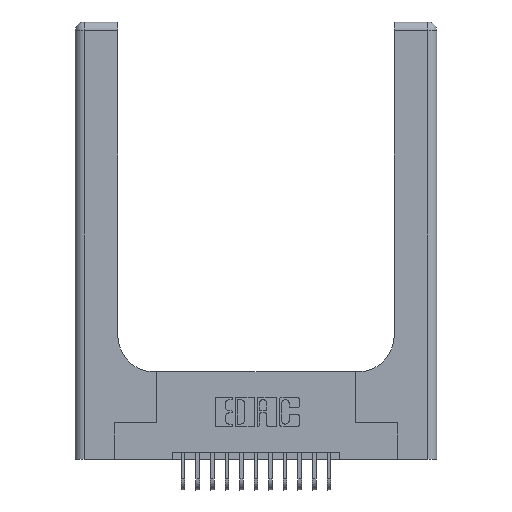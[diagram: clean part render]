
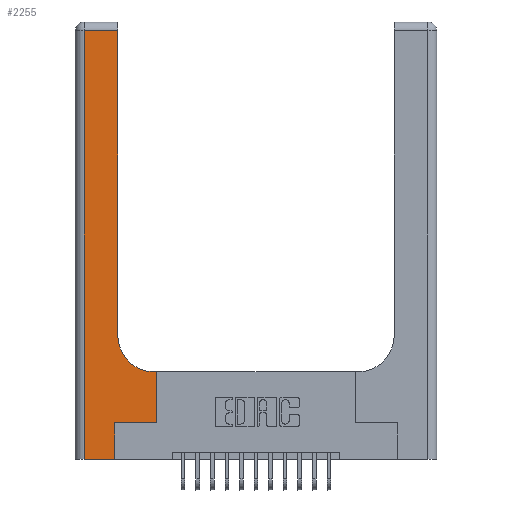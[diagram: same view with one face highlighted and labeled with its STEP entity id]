
A CAD part, top view. The second image highlights one B-rep face of the part: STEP entity #2255.
In plain terms, the highlighted planar face has unit normal (0, 0, 1).
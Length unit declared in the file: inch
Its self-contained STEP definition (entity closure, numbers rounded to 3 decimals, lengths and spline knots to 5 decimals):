
#16 = VECTOR ( 'NONE', #14650, 39.37008 ) ;
#602 = LINE ( 'NONE', #11856, #10853 ) ;
#679 = DIRECTION ( 'NONE',  ( 0., 0., -1. ) ) ;
#1124 = CARTESIAN_POINT ( 'NONE',  ( 0.269, 0., 0.37 ) ) ;
#1543 = DIRECTION ( 'NONE',  ( 0., 1., 0. ) ) ;
#1904 = CARTESIAN_POINT ( 'NONE',  ( 0.5585, 0.6, 0.37 ) ) ;
#1957 = LINE ( 'NONE', #9040, #16 ) ;
#2153 = EDGE_CURVE ( 'NONE', #2332, #11790, #8864, .T. ) ;
#2218 = VECTOR ( 'NONE', #12598, 39.37008 ) ;
#2237 = DIRECTION ( 'NONE',  ( 1., 0., 0. ) ) ;
#2255 = ADVANCED_FACE ( 'NONE', ( #17376 ), #9084, .F. ) ;
#2332 = VERTEX_POINT ( 'NONE', #1904 ) ;
#2705 = LINE ( 'NONE', #9562, #2218 ) ;
#3342 = VERTEX_POINT ( 'NONE', #10067 ) ;
#3783 = VECTOR ( 'NONE', #17413, 39.37008 ) ;
#3848 = EDGE_CURVE ( 'NONE', #3342, #5929, #4271, .T. ) ;
#3990 = ORIENTED_EDGE ( 'NONE', *, *, #2153, .T. ) ;
#4271 = LINE ( 'NONE', #15719, #3783 ) ;
#4307 = CIRCLE ( 'NONE', #9821, 0.25 ) ;
#4372 = DIRECTION ( 'NONE',  ( 0., 0., -1. ) ) ;
#5025 = CARTESIAN_POINT ( 'NONE',  ( 0.06, 2.94, 0.37 ) ) ;
#5256 = ORIENTED_EDGE ( 'NONE', *, *, #3848, .T. ) ;
#5929 = VERTEX_POINT ( 'NONE', #1124 ) ;
#6102 = EDGE_CURVE ( 'NONE', #5929, #15019, #13460, .T. ) ;
#6282 = VERTEX_POINT ( 'NONE', #5025 ) ;
#7884 = EDGE_CURVE ( 'NONE', #10802, #2332, #602, .T. ) ;
#8006 = ORIENTED_EDGE ( 'NONE', *, *, #7884, .T. ) ;
#8408 = LINE ( 'NONE', #17458, #19035 ) ;
#8812 = VERTEX_POINT ( 'NONE', #16460 ) ;
#8864 = LINE ( 'NONE', #18346, #17853 ) ;
#8961 = CARTESIAN_POINT ( 'NONE',  ( 0., 3., 0.37 ) ) ;
#9040 = CARTESIAN_POINT ( 'NONE',  ( 0.06, 3., 0.37 ) ) ;
#9084 = PLANE ( 'NONE',  #9368 ) ;
#9161 = ORIENTED_EDGE ( 'NONE', *, *, #9872, .T. ) ;
#9368 = AXIS2_PLACEMENT_3D ( 'NONE', #8961, #4372, #19662 ) ;
#9562 = CARTESIAN_POINT ( 'NONE',  ( 0., 2.94, 0.37 ) ) ;
#9711 = ORIENTED_EDGE ( 'NONE', *, *, #6102, .T. ) ;
#9805 = CARTESIAN_POINT ( 'NONE',  ( 0.5415, 0.85, 0.37 ) ) ;
#9821 = AXIS2_PLACEMENT_3D ( 'NONE', #9805, #679, #2237 ) ;
#9863 = DIRECTION ( 'NONE',  ( 1., 0., 0. ) ) ;
#9872 = EDGE_CURVE ( 'NONE', #15019, #10802, #8408, .T. ) ;
#10067 = CARTESIAN_POINT ( 'NONE',  ( 0.06, 0., 0.37 ) ) ;
#10802 = VERTEX_POINT ( 'NONE', #13608 ) ;
#10853 = VECTOR ( 'NONE', #13407, 39.37008 ) ;
#10947 = EDGE_CURVE ( 'NONE', #17539, #6282, #2705, .T. ) ;
#11589 = VECTOR ( 'NONE', #1543, 39.37008 ) ;
#11790 = VERTEX_POINT ( 'NONE', #18563 ) ;
#11856 = CARTESIAN_POINT ( 'NONE',  ( 0.5585, 0.25, 0.37 ) ) ;
#12331 = DIRECTION ( 'NONE',  ( -1., 0., 0. ) ) ;
#12598 = DIRECTION ( 'NONE',  ( -1., 0., 0. ) ) ;
#12745 = EDGE_LOOP ( 'NONE', ( #15346, #14539, #19457, #5256, #9711, #9161, #8006, #3990, #13312 ) ) ;
#13312 = ORIENTED_EDGE ( 'NONE', *, *, #15922, .T. ) ;
#13407 = DIRECTION ( 'NONE',  ( 0., 1., 0. ) ) ;
#13460 = LINE ( 'NONE', #19463, #13933 ) ;
#13608 = CARTESIAN_POINT ( 'NONE',  ( 0.5585, 0.25, 0.37 ) ) ;
#13692 = CARTESIAN_POINT ( 'NONE',  ( 0.269, 0.25, 0.37 ) ) ;
#13933 = VECTOR ( 'NONE', #14979, 39.37008 ) ;
#14539 = ORIENTED_EDGE ( 'NONE', *, *, #10947, .T. ) ;
#14650 = DIRECTION ( 'NONE',  ( 0., -1., 0. ) ) ;
#14979 = DIRECTION ( 'NONE',  ( 0., 1., 0. ) ) ;
#15019 = VERTEX_POINT ( 'NONE', #13692 ) ;
#15064 = CARTESIAN_POINT ( 'NONE',  ( 0.2915, 3., 0.37 ) ) ;
#15346 = ORIENTED_EDGE ( 'NONE', *, *, #18222, .T. ) ;
#15719 = CARTESIAN_POINT ( 'NONE',  ( 0., 0., 0.37 ) ) ;
#15922 = EDGE_CURVE ( 'NONE', #11790, #8812, #4307, .T. ) ;
#16460 = CARTESIAN_POINT ( 'NONE',  ( 0.2915, 0.85, 0.37 ) ) ;
#16602 = EDGE_CURVE ( 'NONE', #6282, #3342, #1957, .T. ) ;
#17376 = FACE_OUTER_BOUND ( 'NONE', #12745, .T. ) ;
#17413 = DIRECTION ( 'NONE',  ( 1., 0., 0. ) ) ;
#17458 = CARTESIAN_POINT ( 'NONE',  ( 0.269, 0.25, 0.37 ) ) ;
#17539 = VERTEX_POINT ( 'NONE', #19491 ) ;
#17853 = VECTOR ( 'NONE', #12331, 39.37008 ) ;
#18222 = EDGE_CURVE ( 'NONE', #8812, #17539, #19650, .T. ) ;
#18346 = CARTESIAN_POINT ( 'NONE',  ( 0.2915, 0.6, 0.37 ) ) ;
#18563 = CARTESIAN_POINT ( 'NONE',  ( 0.5415, 0.6, 0.37 ) ) ;
#19035 = VECTOR ( 'NONE', #9863, 39.37008 ) ;
#19457 = ORIENTED_EDGE ( 'NONE', *, *, #16602, .T. ) ;
#19463 = CARTESIAN_POINT ( 'NONE',  ( 0.269, 0., 0.37 ) ) ;
#19491 = CARTESIAN_POINT ( 'NONE',  ( 0.2915, 2.94, 0.37 ) ) ;
#19650 = LINE ( 'NONE', #15064, #11589 ) ;
#19662 = DIRECTION ( 'NONE',  ( -1., 0., 0. ) ) ;
